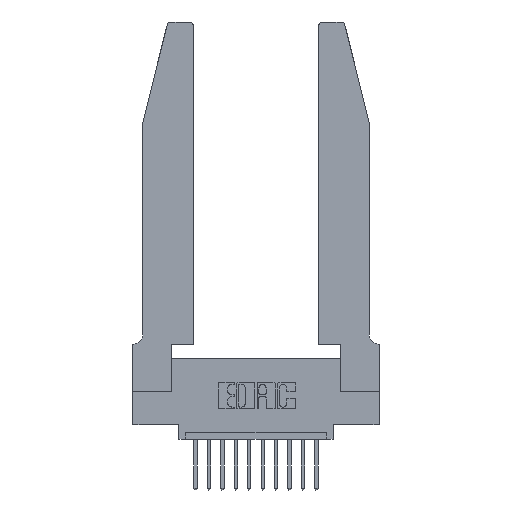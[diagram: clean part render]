
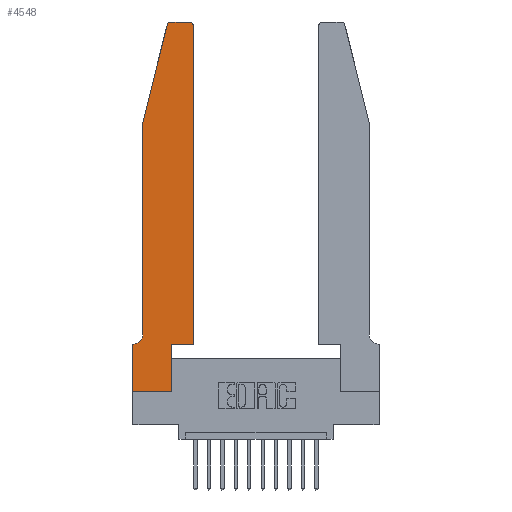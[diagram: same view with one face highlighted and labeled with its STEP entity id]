
A CAD part, top view. The second image highlights one B-rep face of the part: STEP entity #4548.
In plain terms, the highlighted planar face has unit normal (0, 0, 1).
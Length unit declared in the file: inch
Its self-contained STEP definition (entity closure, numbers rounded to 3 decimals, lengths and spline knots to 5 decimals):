
#262 = ORIENTED_EDGE ( 'NONE', *, *, #14025, .T. ) ;
#429 = DIRECTION ( 'NONE',  ( 0., 0., -1. ) ) ;
#452 = EDGE_CURVE ( 'NONE', #3591, #4115, #2732, .T. ) ;
#730 = CARTESIAN_POINT ( 'NONE',  ( 0.2865, 0.35, 0.37 ) ) ;
#841 = VECTOR ( 'NONE', #16666, 39.37008 ) ;
#1110 = AXIS2_PLACEMENT_3D ( 'NONE', #8200, #429, #9458 ) ;
#1181 = CARTESIAN_POINT ( 'NONE',  ( 0.2865, 0.35, 0.37 ) ) ;
#1252 = EDGE_CURVE ( 'NONE', #4115, #4664, #5573, .T. ) ;
#1788 = PLANE ( 'NONE',  #5923 ) ;
#1824 = CARTESIAN_POINT ( 'NONE',  ( 0.4505, 0.35, 0.37 ) ) ;
#1955 = CARTESIAN_POINT ( 'NONE',  ( 0., 0.35, 0.37 ) ) ;
#2141 = CARTESIAN_POINT ( 'NONE',  ( 0., 0., 0.37 ) ) ;
#2265 = EDGE_CURVE ( 'NONE', #8793, #12438, #6780, .T. ) ;
#2732 = LINE ( 'NONE', #1181, #16123 ) ;
#2813 = ORIENTED_EDGE ( 'NONE', *, *, #15509, .T. ) ;
#2848 = AXIS2_PLACEMENT_3D ( 'NONE', #7614, #7514, #13984 ) ;
#2917 = DIRECTION ( 'NONE',  ( -1., 0., 0. ) ) ;
#2983 = LINE ( 'NONE', #11417, #6712 ) ;
#3074 = DIRECTION ( 'NONE',  ( 1., 0., 0. ) ) ;
#3113 = CARTESIAN_POINT ( 'NONE',  ( 0.4505, 0.35, 0.37 ) ) ;
#3465 = CARTESIAN_POINT ( 'NONE',  ( 0., 0., 0.37 ) ) ;
#3591 = VERTEX_POINT ( 'NONE', #8781 ) ;
#3820 = VERTEX_POINT ( 'NONE', #5020 ) ;
#4092 = VERTEX_POINT ( 'NONE', #9833 ) ;
#4115 = VERTEX_POINT ( 'NONE', #730 ) ;
#4262 = EDGE_CURVE ( 'NONE', #5590, #9754, #4689, .T. ) ;
#4447 = DIRECTION ( 'NONE',  ( 0., 1., 0. ) ) ;
#4472 = EDGE_CURVE ( 'NONE', #4664, #5610, #11764, .T. ) ;
#4498 = EDGE_CURVE ( 'NONE', #4588, #4092, #4669, .T. ) ;
#4548 = ADVANCED_FACE ( 'NONE', ( #14177 ), #1788, .T. ) ;
#4588 = VERTEX_POINT ( 'NONE', #10352 ) ;
#4640 = EDGE_CURVE ( 'NONE', #3820, #8793, #6943, .T. ) ;
#4664 = VERTEX_POINT ( 'NONE', #15638 ) ;
#4669 = CIRCLE ( 'NONE', #8749, 0.03 ) ;
#4689 = LINE ( 'NONE', #5083, #841 ) ;
#5020 = CARTESIAN_POINT ( 'NONE',  ( 0.0755, 2., 0.37 ) ) ;
#5083 = CARTESIAN_POINT ( 'NONE',  ( 0., 0., 0.37 ) ) ;
#5115 = ORIENTED_EDGE ( 'NONE', *, *, #12875, .T. ) ;
#5520 = EDGE_CURVE ( 'NONE', #4092, #3820, #2983, .T. ) ;
#5572 = ORIENTED_EDGE ( 'NONE', *, *, #1252, .T. ) ;
#5573 = LINE ( 'NONE', #1824, #13460 ) ;
#5590 = VERTEX_POINT ( 'NONE', #13520 ) ;
#5610 = VERTEX_POINT ( 'NONE', #11241 ) ;
#5919 = DIRECTION ( 'NONE',  ( 1., 0., 0. ) ) ;
#5923 = AXIS2_PLACEMENT_3D ( 'NONE', #1955, #12320, #3074 ) ;
#6418 = ORIENTED_EDGE ( 'NONE', *, *, #452, .T. ) ;
#6490 = DIRECTION ( 'NONE',  ( 0., 1., 0. ) ) ;
#6712 = VECTOR ( 'NONE', #12749, 39.37008 ) ;
#6780 = CIRCLE ( 'NONE', #1110, 0.07 ) ;
#6942 = EDGE_CURVE ( 'NONE', #15478, #4588, #14686, .T. ) ;
#6943 = LINE ( 'NONE', #8820, #10910 ) ;
#7282 = VECTOR ( 'NONE', #15375, 39.37008 ) ;
#7386 = ORIENTED_EDGE ( 'NONE', *, *, #4262, .T. ) ;
#7514 = DIRECTION ( 'NONE',  ( 0., 0., 1. ) ) ;
#7614 = CARTESIAN_POINT ( 'NONE',  ( 0.4205, 2.72, 0.37 ) ) ;
#8200 = CARTESIAN_POINT ( 'NONE',  ( 0.0055, 0.42, 0.37 ) ) ;
#8404 = DIRECTION ( 'NONE',  ( 0., 0., 1. ) ) ;
#8671 = ORIENTED_EDGE ( 'NONE', *, *, #6942, .T. ) ;
#8749 = AXIS2_PLACEMENT_3D ( 'NONE', #15104, #8404, #5919 ) ;
#8750 = VECTOR ( 'NONE', #4447, 39.37008 ) ;
#8781 = CARTESIAN_POINT ( 'NONE',  ( 0.2865, 0., 0.37 ) ) ;
#8793 = VERTEX_POINT ( 'NONE', #12042 ) ;
#8808 = VECTOR ( 'NONE', #2917, 39.37008 ) ;
#8820 = CARTESIAN_POINT ( 'NONE',  ( 0.0755, 2., 0.37 ) ) ;
#9317 = ORIENTED_EDGE ( 'NONE', *, *, #5520, .T. ) ;
#9458 = DIRECTION ( 'NONE',  ( -1., 0., 0. ) ) ;
#9754 = VERTEX_POINT ( 'NONE', #3465 ) ;
#9833 = CARTESIAN_POINT ( 'NONE',  ( 0.25487, 2.72718, 0.37 ) ) ;
#10067 = LINE ( 'NONE', #2141, #7282 ) ;
#10352 = CARTESIAN_POINT ( 'NONE',  ( 0.284, 2.75, 0.37 ) ) ;
#10857 = DIRECTION ( 'NONE',  ( 1., 0., 0. ) ) ;
#10910 = VECTOR ( 'NONE', #15121, 39.37008 ) ;
#11241 = CARTESIAN_POINT ( 'NONE',  ( 0.4505, 2.72, 0.37 ) ) ;
#11417 = CARTESIAN_POINT ( 'NONE',  ( 0.0755, 2., 0.37 ) ) ;
#11651 = ORIENTED_EDGE ( 'NONE', *, *, #2265, .T. ) ;
#11764 = LINE ( 'NONE', #3113, #8750 ) ;
#11782 = CARTESIAN_POINT ( 'NONE',  ( 0.4205, 2.75, 0.37 ) ) ;
#11961 = ORIENTED_EDGE ( 'NONE', *, *, #4472, .T. ) ;
#12042 = CARTESIAN_POINT ( 'NONE',  ( 0.0755, 0.42, 0.37 ) ) ;
#12320 = DIRECTION ( 'NONE',  ( 0., 0., 1. ) ) ;
#12438 = VERTEX_POINT ( 'NONE', #13795 ) ;
#12749 = DIRECTION ( 'NONE',  ( -0.239, -0.971, 0. ) ) ;
#12875 = EDGE_CURVE ( 'NONE', #9754, #3591, #10067, .T. ) ;
#13016 = CARTESIAN_POINT ( 'NONE',  ( 0.2605, 2.75, 0.37 ) ) ;
#13460 = VECTOR ( 'NONE', #10857, 39.37008 ) ;
#13520 = CARTESIAN_POINT ( 'NONE',  ( 0., 0.35, 0.37 ) ) ;
#13527 = ORIENTED_EDGE ( 'NONE', *, *, #4640, .T. ) ;
#13795 = CARTESIAN_POINT ( 'NONE',  ( 0.0055, 0.35, 0.37 ) ) ;
#13984 = DIRECTION ( 'NONE',  ( 1., 0., 0. ) ) ;
#14025 = EDGE_CURVE ( 'NONE', #5610, #15478, #16503, .T. ) ;
#14177 = FACE_OUTER_BOUND ( 'NONE', #15109, .T. ) ;
#14422 = CARTESIAN_POINT ( 'NONE',  ( 0.0755, 0.35, 0.37 ) ) ;
#14686 = LINE ( 'NONE', #13016, #16719 ) ;
#15104 = CARTESIAN_POINT ( 'NONE',  ( 0.284, 2.72, 0.37 ) ) ;
#15109 = EDGE_LOOP ( 'NONE', ( #8671, #15127, #9317, #13527, #11651, #2813, #7386, #5115, #6418, #5572, #11961, #262 ) ) ;
#15121 = DIRECTION ( 'NONE',  ( 0., -1., 0. ) ) ;
#15127 = ORIENTED_EDGE ( 'NONE', *, *, #4498, .T. ) ;
#15375 = DIRECTION ( 'NONE',  ( 1., 0., 0. ) ) ;
#15478 = VERTEX_POINT ( 'NONE', #11782 ) ;
#15509 = EDGE_CURVE ( 'NONE', #12438, #5590, #15664, .T. ) ;
#15638 = CARTESIAN_POINT ( 'NONE',  ( 0.4505, 0.35, 0.37 ) ) ;
#15664 = LINE ( 'NONE', #14422, #8808 ) ;
#16123 = VECTOR ( 'NONE', #6490, 39.37008 ) ;
#16162 = DIRECTION ( 'NONE',  ( -1., 0., 0. ) ) ;
#16503 = CIRCLE ( 'NONE', #2848, 0.03 ) ;
#16666 = DIRECTION ( 'NONE',  ( 0., -1., 0. ) ) ;
#16719 = VECTOR ( 'NONE', #16162, 39.37008 ) ;
